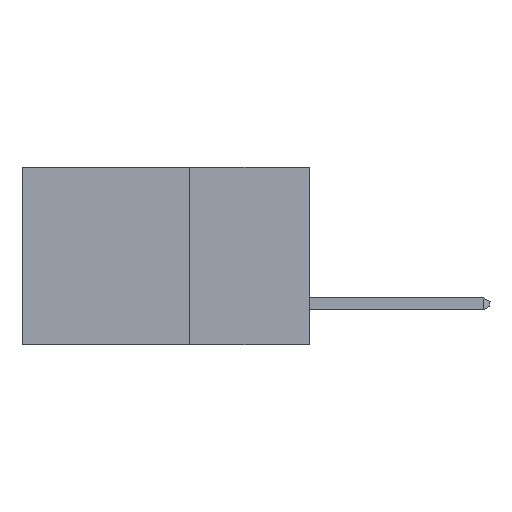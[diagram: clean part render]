
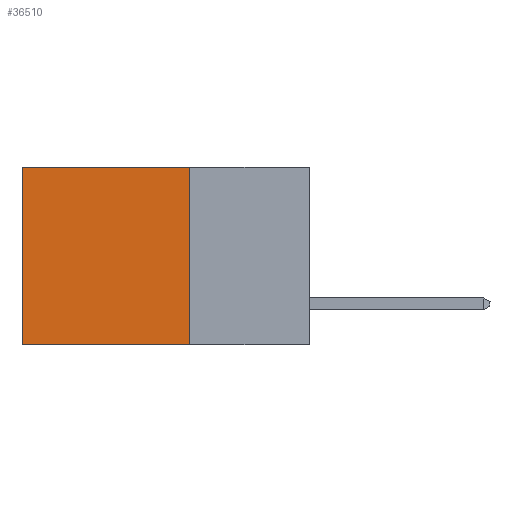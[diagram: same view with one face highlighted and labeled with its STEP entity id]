
A CAD part, left-side view. The second image highlights one B-rep face of the part: STEP entity #36510.
In plain terms, the highlighted planar face has unit normal (-1, 0, 0).
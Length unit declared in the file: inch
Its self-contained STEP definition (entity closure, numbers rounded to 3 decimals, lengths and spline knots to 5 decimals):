
#1755 = DIRECTION ( 'NONE',  ( 1., 0., 0. ) ) ;
#1956 = CARTESIAN_POINT ( 'NONE',  ( 0.2875, 0.25, 0. ) ) ;
#2331 = LINE ( 'NONE', #15876, #13262 ) ;
#2766 = CARTESIAN_POINT ( 'NONE',  ( 0.2875, 0.25, -0.37 ) ) ;
#4559 = ORIENTED_EDGE ( 'NONE', *, *, #35623, .T. ) ;
#5604 = EDGE_CURVE ( 'NONE', #9499, #26253, #13742, .T. ) ;
#5622 = LINE ( 'NONE', #2766, #24120 ) ;
#7590 = DIRECTION ( 'NONE',  ( 0., 1., 0. ) ) ;
#8977 = AXIS2_PLACEMENT_3D ( 'NONE', #1956, #1755, #15304 ) ;
#9035 = VERTEX_POINT ( 'NONE', #20165 ) ;
#9499 = VERTEX_POINT ( 'NONE', #13576 ) ;
#10633 = EDGE_LOOP ( 'NONE', ( #39283, #22219, #20978, #4559 ) ) ;
#11083 = CARTESIAN_POINT ( 'NONE',  ( 0.2875, 0.25, 0. ) ) ;
#12697 = VECTOR ( 'NONE', #27494, 39.37008 ) ;
#13262 = VECTOR ( 'NONE', #22650, 39.37008 ) ;
#13576 = CARTESIAN_POINT ( 'NONE',  ( 0.2875, 0.25, 0. ) ) ;
#13742 = LINE ( 'NONE', #14172, #12697 ) ;
#14172 = CARTESIAN_POINT ( 'NONE',  ( 0.2875, 0.25, 0. ) ) ;
#15304 = DIRECTION ( 'NONE',  ( 0., 0., -1. ) ) ;
#15876 = CARTESIAN_POINT ( 'NONE',  ( 0.2875, 0.6, 0. ) ) ;
#16949 = CARTESIAN_POINT ( 'NONE',  ( 0.2875, 0.6, 0. ) ) ;
#18370 = FACE_OUTER_BOUND ( 'NONE', #10633, .T. ) ;
#20165 = CARTESIAN_POINT ( 'NONE',  ( 0.2875, 0.6, -0.37 ) ) ;
#20978 = ORIENTED_EDGE ( 'NONE', *, *, #5604, .F. ) ;
#22219 = ORIENTED_EDGE ( 'NONE', *, *, #31154, .F. ) ;
#22259 = VERTEX_POINT ( 'NONE', #16949 ) ;
#22650 = DIRECTION ( 'NONE',  ( 0., 0., -1. ) ) ;
#24120 = VECTOR ( 'NONE', #29010, 39.37008 ) ;
#26253 = VERTEX_POINT ( 'NONE', #41632 ) ;
#27494 = DIRECTION ( 'NONE',  ( 0., 0., -1. ) ) ;
#29010 = DIRECTION ( 'NONE',  ( 0., 1., 0. ) ) ;
#31154 = EDGE_CURVE ( 'NONE', #26253, #9035, #5622, .T. ) ;
#31900 = PLANE ( 'NONE',  #8977 ) ;
#35623 = EDGE_CURVE ( 'NONE', #9499, #22259, #41004, .T. ) ;
#36510 = ADVANCED_FACE ( 'NONE', ( #18370 ), #31900, .F. ) ;
#39283 = ORIENTED_EDGE ( 'NONE', *, *, #43151, .T. ) ;
#41004 = LINE ( 'NONE', #11083, #43117 ) ;
#41632 = CARTESIAN_POINT ( 'NONE',  ( 0.2875, 0.25, -0.37 ) ) ;
#43117 = VECTOR ( 'NONE', #7590, 39.37008 ) ;
#43151 = EDGE_CURVE ( 'NONE', #22259, #9035, #2331, .T. ) ;
